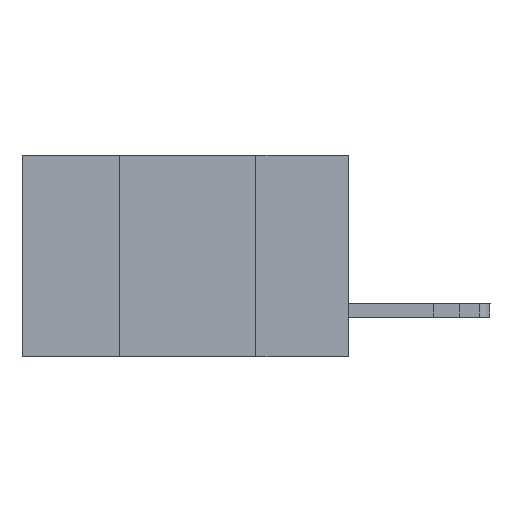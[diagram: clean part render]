
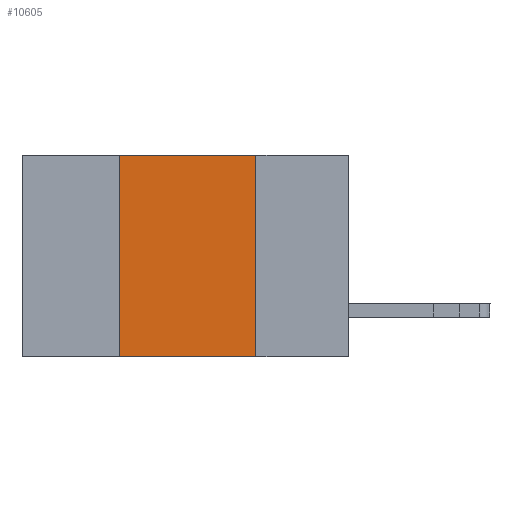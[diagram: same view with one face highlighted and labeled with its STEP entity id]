
A CAD part, left-side view. The second image highlights one B-rep face of the part: STEP entity #10605.
In plain terms, the highlighted planar face has unit normal (-1, 0, 0).
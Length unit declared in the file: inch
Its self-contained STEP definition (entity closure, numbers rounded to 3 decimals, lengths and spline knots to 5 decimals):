
#126 = CARTESIAN_POINT ( 'NONE',  ( 0., 0.6, 0. ) ) ;
#434 = PLANE ( 'NONE',  #8187 ) ;
#1062 = VERTEX_POINT ( 'NONE', #19490 ) ;
#1167 = VERTEX_POINT ( 'NONE', #18239 ) ;
#1526 = EDGE_CURVE ( 'NONE', #1062, #16164, #10056, .T. ) ;
#2100 = CARTESIAN_POINT ( 'NONE',  ( 0., 0.6, -0.37 ) ) ;
#2355 = CARTESIAN_POINT ( 'NONE',  ( 0., 0.42, 0. ) ) ;
#3096 = ORIENTED_EDGE ( 'NONE', *, *, #15479, .F. ) ;
#4388 = ORIENTED_EDGE ( 'NONE', *, *, #9353, .F. ) ;
#4671 = VECTOR ( 'NONE', #8487, 39.37008 ) ;
#4930 = FACE_OUTER_BOUND ( 'NONE', #19775, .T. ) ;
#7437 = VECTOR ( 'NONE', #9540, 39.37008 ) ;
#7701 = EDGE_CURVE ( 'NONE', #1062, #15388, #13094, .T. ) ;
#7982 = DIRECTION ( 'NONE',  ( 1., 0., 0. ) ) ;
#8187 = AXIS2_PLACEMENT_3D ( 'NONE', #126, #7982, #17909 ) ;
#8402 = CARTESIAN_POINT ( 'NONE',  ( 0., 0.42, -0.37 ) ) ;
#8470 = LINE ( 'NONE', #17882, #10028 ) ;
#8487 = DIRECTION ( 'NONE',  ( 0., -1., 0. ) ) ;
#9353 = EDGE_CURVE ( 'NONE', #15388, #1167, #8470, .T. ) ;
#9540 = DIRECTION ( 'NONE',  ( 0., 0., -1. ) ) ;
#10028 = VECTOR ( 'NONE', #13371, 39.37008 ) ;
#10056 = LINE ( 'NONE', #2100, #4671 ) ;
#10136 = ORIENTED_EDGE ( 'NONE', *, *, #7701, .F. ) ;
#10605 = ADVANCED_FACE ( 'NONE', ( #4930 ), #434, .F. ) ;
#12073 = LINE ( 'NONE', #12571, #7437 ) ;
#12571 = CARTESIAN_POINT ( 'NONE',  ( 0., 0.17, -0.37 ) ) ;
#13094 = LINE ( 'NONE', #8402, #13871 ) ;
#13371 = DIRECTION ( 'NONE',  ( 0., -1., 0. ) ) ;
#13871 = VECTOR ( 'NONE', #14750, 39.37008 ) ;
#14750 = DIRECTION ( 'NONE',  ( 0., 0., 1. ) ) ;
#15388 = VERTEX_POINT ( 'NONE', #2355 ) ;
#15479 = EDGE_CURVE ( 'NONE', #1167, #16164, #12073, .T. ) ;
#16164 = VERTEX_POINT ( 'NONE', #17614 ) ;
#17614 = CARTESIAN_POINT ( 'NONE',  ( 0., 0.17, -0.37 ) ) ;
#17882 = CARTESIAN_POINT ( 'NONE',  ( 0., 0.6, 0. ) ) ;
#17909 = DIRECTION ( 'NONE',  ( 0., 0., -1. ) ) ;
#18239 = CARTESIAN_POINT ( 'NONE',  ( 0., 0.17, 0. ) ) ;
#19490 = CARTESIAN_POINT ( 'NONE',  ( 0., 0.42, -0.37 ) ) ;
#19559 = ORIENTED_EDGE ( 'NONE', *, *, #1526, .T. ) ;
#19775 = EDGE_LOOP ( 'NONE', ( #3096, #4388, #10136, #19559 ) ) ;
